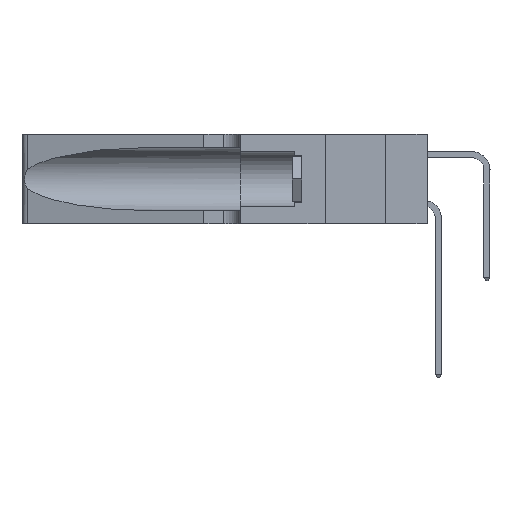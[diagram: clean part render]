
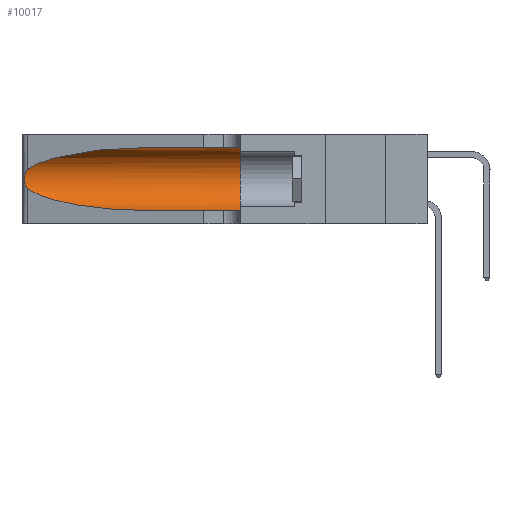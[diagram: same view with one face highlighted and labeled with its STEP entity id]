
A CAD part, left-side view. The second image highlights one B-rep face of the part: STEP entity #10017.
In plain terms, the highlighted cylindrical face has radius 3.308 mm (diameter 6.617 mm), a partial arc.
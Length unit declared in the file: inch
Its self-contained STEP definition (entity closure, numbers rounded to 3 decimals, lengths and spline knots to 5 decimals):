
#434 = AXIS2_PLACEMENT_3D ( 'NONE', #22881, #12100, #754 ) ;
#462 = CARTESIAN_POINT ( 'NONE',  ( 0.25787, 1.23484, 0.2124 ) ) ;
#754 = DIRECTION ( 'NONE',  ( 0., 0., 1. ) ) ;
#1122 = EDGE_CURVE ( 'NONE', #18720, #21393, #13243, .T. ) ;
#1197 = VECTOR ( 'NONE', #7072, 39.37008 ) ;
#1786 = LINE ( 'NONE', #5170, #1197 ) ;
#1875 = VERTEX_POINT ( 'NONE', #15903 ) ;
#2106 = ORIENTED_EDGE ( 'NONE', *, *, #3608, .T. ) ;
#2230 = ORIENTED_EDGE ( 'NONE', *, *, #1122, .T. ) ;
#2388 = CARTESIAN_POINT ( 'NONE',  ( 0.26018, 1.23835, 0.19895 ) ) ;
#2748 = CARTESIAN_POINT ( 'NONE',  ( 0.18966, 0.96281, 0.05475 ) ) ;
#3230 = CARTESIAN_POINT ( 'NONE',  ( 0.25487, 1.22718, 0.14631 ) ) ;
#3608 = EDGE_CURVE ( 'NONE', #21393, #21831, #17288, .T. ) ;
#4306 = CARTESIAN_POINT ( 'NONE',  ( 0.26075, 1.23896, 0.178 ) ) ;
#4647 = CARTESIAN_POINT ( 'NONE',  ( 0.25487, 1.22718, 0.22369 ) ) ;
#5105 = CARTESIAN_POINT ( 'NONE',  ( 0.1305, 1.61858, 0.31525 ) ) ;
#5170 = CARTESIAN_POINT ( 'NONE',  ( 0.1305, 1.61858, 0.05475 ) ) ;
#5621 = EDGE_CURVE ( 'NONE', #21831, #16774, #9215, .T. ) ;
#6054 = CARTESIAN_POINT ( 'NONE',  ( 0.25555, 1.22994, 0.2215 ) ) ;
#6223 = CARTESIAN_POINT ( 'NONE',  ( 0.25856, 1.23593, 0.16098 ) ) ;
#6964 = CYLINDRICAL_SURFACE ( 'NONE', #15640, 0.13025 ) ;
#7072 = DIRECTION ( 'NONE',  ( 0., -1., 0. ) ) ;
#7622 = ORIENTED_EDGE ( 'NONE', *, *, #13325, .T. ) ;
#7927 = DIRECTION ( 'NONE',  ( 0., -1., 0. ) ) ;
#8031 = EDGE_CURVE ( 'NONE', #18720, #1875, #9435, .T. ) ;
#8096 = CARTESIAN_POINT ( 'NONE',  ( 0.25639, 1.23186, 0.15144 ) ) ;
#9215 =( BOUNDED_CURVE ( )  B_SPLINE_CURVE ( 3, ( #12178, #13992, #2748, #15795 ),
 .UNSPECIFIED., .F., .F. ) 
 B_SPLINE_CURVE_WITH_KNOTS ( ( 4, 4 ),
 ( 3.44316, 4.71239 ),
 .UNSPECIFIED. ) 
 CURVE ( )  GEOMETRIC_REPRESENTATION_ITEM ( )  RATIONAL_B_SPLINE_CURVE ( ( 1., 0.87, 0.87, 1. ) ) 
 REPRESENTATION_ITEM ( '' )  );
#9435 = LINE ( 'NONE', #5105, #13791 ) ;
#9894 = CIRCLE ( 'NONE', #434, 0.13025 ) ;
#10016 = CARTESIAN_POINT ( 'NONE',  ( 0.25487, 1.22718, 0.14631 ) ) ;
#10017 = ADVANCED_FACE ( 'NONE', ( #13116 ), #6964, .F. ) ;
#10814 = EDGE_CURVE ( 'NONE', #1875, #14180, #9894, .T. ) ;
#11812 = CARTESIAN_POINT ( 'NONE',  ( 0.25639, 1.23184, 0.21858 ) ) ;
#12100 = DIRECTION ( 'NONE',  ( 0., 1., 0. ) ) ;
#12169 = CARTESIAN_POINT ( 'NONE',  ( 0.18966, 0.96281, 0.31525 ) ) ;
#12178 = CARTESIAN_POINT ( 'NONE',  ( 0.25487, 1.22718, 0.14631 ) ) ;
#12244 = ORIENTED_EDGE ( 'NONE', *, *, #5621, .T. ) ;
#13116 = FACE_OUTER_BOUND ( 'NONE', #19370, .T. ) ;
#13243 =( BOUNDED_CURVE ( )  B_SPLINE_CURVE ( 3, ( #19332, #12169, #22930, #4647 ),
 .UNSPECIFIED., .F., .F. ) 
 B_SPLINE_CURVE_WITH_KNOTS ( ( 4, 4 ),
 ( 1.5708, 2.84003 ),
 .UNSPECIFIED. ) 
 CURVE ( )  GEOMETRIC_REPRESENTATION_ITEM ( )  RATIONAL_B_SPLINE_CURVE ( ( 1., 0.87, 0.87, 1. ) ) 
 REPRESENTATION_ITEM ( '' )  );
#13325 = EDGE_CURVE ( 'NONE', #16774, #14180, #1786, .T. ) ;
#13579 = CARTESIAN_POINT ( 'NONE',  ( 0.25487, 1.22718, 0.22369 ) ) ;
#13651 = CARTESIAN_POINT ( 'NONE',  ( 0.25854, 1.2359, 0.20912 ) ) ;
#13712 = ORIENTED_EDGE ( 'NONE', *, *, #10814, .F. ) ;
#13791 = VECTOR ( 'NONE', #14491, 39.37008 ) ;
#13992 = CARTESIAN_POINT ( 'NONE',  ( 0.2373, 1.15595, 0.08982 ) ) ;
#14180 = VERTEX_POINT ( 'NONE', #16781 ) ;
#14491 = DIRECTION ( 'NONE',  ( 0., -1., 0. ) ) ;
#15457 = CARTESIAN_POINT ( 'NONE',  ( 0.26075, 1.23896, 0.19203 ) ) ;
#15640 = AXIS2_PLACEMENT_3D ( 'NONE', #18897, #7927, #20721 ) ;
#15795 = CARTESIAN_POINT ( 'NONE',  ( 0.1305, 0.72297, 0.05475 ) ) ;
#15903 = CARTESIAN_POINT ( 'NONE',  ( 0.1305, 0.35, 0.31525 ) ) ;
#16774 = VERTEX_POINT ( 'NONE', #21288 ) ;
#16781 = CARTESIAN_POINT ( 'NONE',  ( 0.1305, 0.35, 0.05475 ) ) ;
#17257 = CARTESIAN_POINT ( 'NONE',  ( 0.26017, 1.23833, 0.17102 ) ) ;
#17288 = B_SPLINE_CURVE_WITH_KNOTS ( 'NONE', 3,
 ( #13579, #6054, #11812, #462, #13651, #2388, #15457, #4306, #17257, #6223, #19065, #8096, #20891, #10016 ),
 .UNSPECIFIED., .F., .F.,
 ( 4, 2, 2, 2, 2, 2, 4 ),
 ( 0., 0.00027, 0.00053, 0.00107, 0.0016, 0.00187, 0.00214 ),
 .UNSPECIFIED. ) ;
#18720 = VERTEX_POINT ( 'NONE', #19851 ) ;
#18897 = CARTESIAN_POINT ( 'NONE',  ( 0.1305, 1.61858, 0.185 ) ) ;
#19065 = CARTESIAN_POINT ( 'NONE',  ( 0.25789, 1.23486, 0.15765 ) ) ;
#19304 = ORIENTED_EDGE ( 'NONE', *, *, #8031, .F. ) ;
#19332 = CARTESIAN_POINT ( 'NONE',  ( 0.1305, 0.72297, 0.31525 ) ) ;
#19370 = EDGE_LOOP ( 'NONE', ( #2230, #2106, #12244, #7622, #13712, #19304 ) ) ;
#19851 = CARTESIAN_POINT ( 'NONE',  ( 0.1305, 0.72297, 0.31525 ) ) ;
#20721 = DIRECTION ( 'NONE',  ( 0., 0., -1. ) ) ;
#20891 = CARTESIAN_POINT ( 'NONE',  ( 0.25555, 1.22993, 0.14849 ) ) ;
#21185 = CARTESIAN_POINT ( 'NONE',  ( 0.25487, 1.22718, 0.22369 ) ) ;
#21288 = CARTESIAN_POINT ( 'NONE',  ( 0.1305, 0.72297, 0.05475 ) ) ;
#21393 = VERTEX_POINT ( 'NONE', #21185 ) ;
#21831 = VERTEX_POINT ( 'NONE', #3230 ) ;
#22881 = CARTESIAN_POINT ( 'NONE',  ( 0.1305, 0.35, 0.185 ) ) ;
#22930 = CARTESIAN_POINT ( 'NONE',  ( 0.2373, 1.15595, 0.28018 ) ) ;
